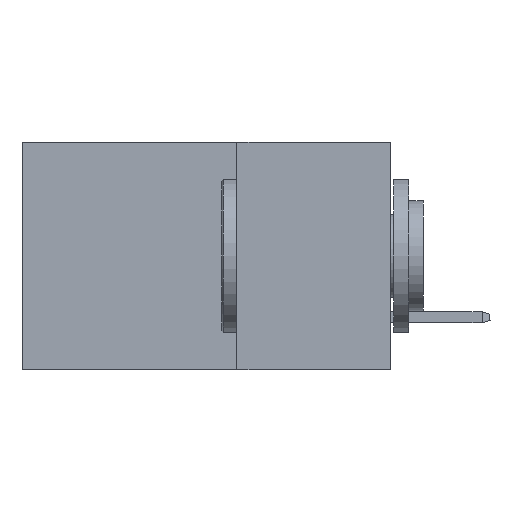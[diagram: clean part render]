
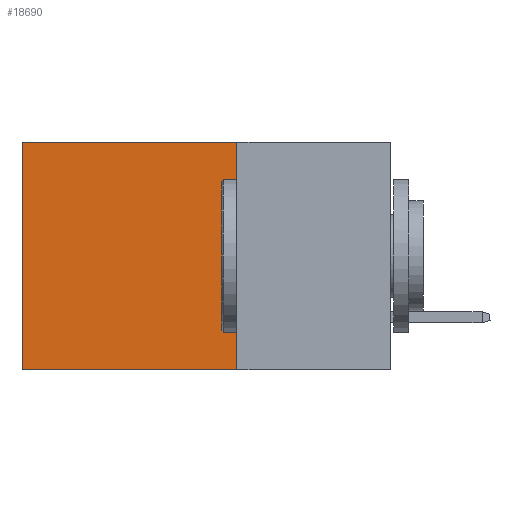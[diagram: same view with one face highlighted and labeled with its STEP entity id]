
A CAD part, left-side view. The second image highlights one B-rep face of the part: STEP entity #18690.
In plain terms, the highlighted planar face has unit normal (-1, 0, 0).
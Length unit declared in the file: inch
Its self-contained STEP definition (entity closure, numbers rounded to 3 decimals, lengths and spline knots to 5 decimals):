
#682 = FACE_OUTER_BOUND ( 'NONE', #35641, .T. ) ;
#1787 = ORIENTED_EDGE ( 'NONE', *, *, #50286, .F. ) ;
#1948 = DIRECTION ( 'NONE',  ( 0., 1., 0. ) ) ;
#1958 = CARTESIAN_POINT ( 'NONE',  ( 0.2875, 0.6, -0.37 ) ) ;
#4218 = LINE ( 'NONE', #25495, #27017 ) ;
#5586 = CARTESIAN_POINT ( 'NONE',  ( 0.2875, 0.25, -0.37 ) ) ;
#5840 = CARTESIAN_POINT ( 'NONE',  ( 0.2875, 0.25, 0. ) ) ;
#6709 = VERTEX_POINT ( 'NONE', #5840 ) ;
#7288 = VECTOR ( 'NONE', #42743, 39.37008 ) ;
#8829 = VERTEX_POINT ( 'NONE', #1958 ) ;
#11046 = CARTESIAN_POINT ( 'NONE',  ( 0.2875, 0.25, 0. ) ) ;
#13057 = EDGE_CURVE ( 'NONE', #6709, #49132, #36204, .T. ) ;
#13625 = ORIENTED_EDGE ( 'NONE', *, *, #14995, .T. ) ;
#14995 = EDGE_CURVE ( 'NONE', #22115, #8829, #29262, .T. ) ;
#15538 = CARTESIAN_POINT ( 'NONE',  ( 0.2875, 0.25, 0. ) ) ;
#17158 = LINE ( 'NONE', #11046, #7288 ) ;
#18690 = ADVANCED_FACE ( 'NONE', ( #682 ), #27186, .F. ) ;
#20473 = DIRECTION ( 'NONE',  ( 1., 0., 0. ) ) ;
#22115 = VERTEX_POINT ( 'NONE', #23993 ) ;
#23154 = VECTOR ( 'NONE', #42875, 39.37008 ) ;
#23993 = CARTESIAN_POINT ( 'NONE',  ( 0.2875, 0.6, 0. ) ) ;
#24601 = VECTOR ( 'NONE', #42922, 39.37008 ) ;
#25495 = CARTESIAN_POINT ( 'NONE',  ( 0.2875, 0.25, -0.37 ) ) ;
#27017 = VECTOR ( 'NONE', #1948, 39.37008 ) ;
#27186 = PLANE ( 'NONE',  #31276 ) ;
#27463 = EDGE_CURVE ( 'NONE', #6709, #22115, #17158, .T. ) ;
#29262 = LINE ( 'NONE', #43041, #23154 ) ;
#30813 = ORIENTED_EDGE ( 'NONE', *, *, #13057, .F. ) ;
#31276 = AXIS2_PLACEMENT_3D ( 'NONE', #15538, #20473, #43582 ) ;
#35641 = EDGE_LOOP ( 'NONE', ( #13625, #1787, #30813, #43566 ) ) ;
#36204 = LINE ( 'NONE', #46535, #24601 ) ;
#42743 = DIRECTION ( 'NONE',  ( 0., 1., 0. ) ) ;
#42875 = DIRECTION ( 'NONE',  ( 0., 0., -1. ) ) ;
#42922 = DIRECTION ( 'NONE',  ( 0., 0., -1. ) ) ;
#43041 = CARTESIAN_POINT ( 'NONE',  ( 0.2875, 0.6, 0. ) ) ;
#43566 = ORIENTED_EDGE ( 'NONE', *, *, #27463, .T. ) ;
#43582 = DIRECTION ( 'NONE',  ( 0., 0., -1. ) ) ;
#46535 = CARTESIAN_POINT ( 'NONE',  ( 0.2875, 0.25, 0. ) ) ;
#49132 = VERTEX_POINT ( 'NONE', #5586 ) ;
#50286 = EDGE_CURVE ( 'NONE', #49132, #8829, #4218, .T. ) ;
